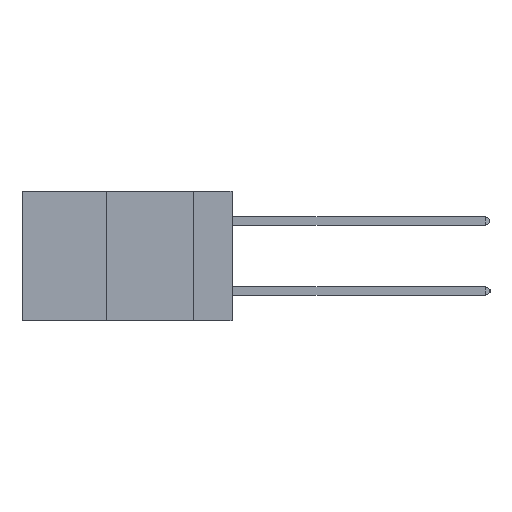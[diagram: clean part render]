
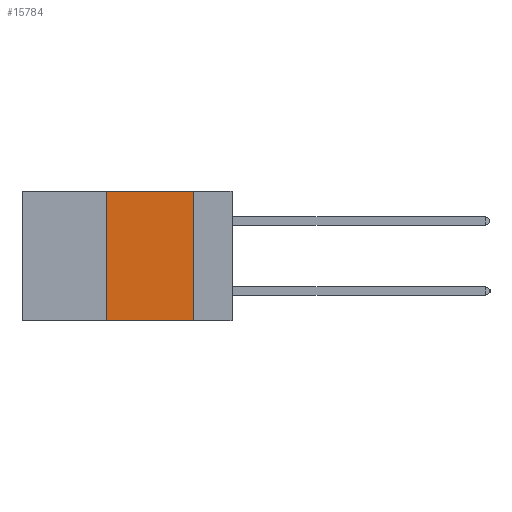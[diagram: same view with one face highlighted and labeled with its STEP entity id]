
A CAD part, left-side view. The second image highlights one B-rep face of the part: STEP entity #15784.
In plain terms, the highlighted planar face has unit normal (-1, 0, 0).
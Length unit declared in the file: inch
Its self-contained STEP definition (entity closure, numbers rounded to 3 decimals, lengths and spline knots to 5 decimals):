
#102 = DIRECTION ( 'NONE',  ( 0., 0., 1. ) ) ;
#830 = DIRECTION ( 'NONE',  ( 0., 0., -1. ) ) ;
#1790 = CARTESIAN_POINT ( 'NONE',  ( 0., 0.11, 0. ) ) ;
#1828 = VERTEX_POINT ( 'NONE', #8338 ) ;
#2219 = CARTESIAN_POINT ( 'NONE',  ( 0., 0.11, -0.37 ) ) ;
#2530 = DIRECTION ( 'NONE',  ( 1., 0., 0. ) ) ;
#2854 = PLANE ( 'NONE',  #9148 ) ;
#3167 = CARTESIAN_POINT ( 'NONE',  ( 0., 0.36, 0. ) ) ;
#4403 = DIRECTION ( 'NONE',  ( 0., 0., -1. ) ) ;
#4586 = ORIENTED_EDGE ( 'NONE', *, *, #15223, .F. ) ;
#4916 = EDGE_CURVE ( 'NONE', #12508, #11015, #20053, .T. ) ;
#5599 = LINE ( 'NONE', #16658, #7349 ) ;
#6593 = CARTESIAN_POINT ( 'NONE',  ( 0., 0.6, 0. ) ) ;
#7247 = DIRECTION ( 'NONE',  ( 0., -1., 0. ) ) ;
#7349 = VECTOR ( 'NONE', #7247, 39.37008 ) ;
#8008 = VECTOR ( 'NONE', #102, 39.37008 ) ;
#8338 = CARTESIAN_POINT ( 'NONE',  ( 0., 0.36, -0.37 ) ) ;
#8354 = VECTOR ( 'NONE', #830, 39.37008 ) ;
#9148 = AXIS2_PLACEMENT_3D ( 'NONE', #6593, #2530, #4403 ) ;
#9599 = ORIENTED_EDGE ( 'NONE', *, *, #10301, .F. ) ;
#10095 = LINE ( 'NONE', #23044, #8354 ) ;
#10301 = EDGE_CURVE ( 'NONE', #1828, #12508, #21917, .T. ) ;
#11015 = VERTEX_POINT ( 'NONE', #1790 ) ;
#11922 = VECTOR ( 'NONE', #23773, 39.37008 ) ;
#12042 = EDGE_CURVE ( 'NONE', #1828, #23139, #5599, .T. ) ;
#12508 = VERTEX_POINT ( 'NONE', #3167 ) ;
#15223 = EDGE_CURVE ( 'NONE', #11015, #23139, #10095, .T. ) ;
#15784 = ADVANCED_FACE ( 'NONE', ( #19367 ), #2854, .F. ) ;
#16475 = CARTESIAN_POINT ( 'NONE',  ( 0., 0.6, 0. ) ) ;
#16564 = EDGE_LOOP ( 'NONE', ( #4586, #17260, #9599, #19724 ) ) ;
#16658 = CARTESIAN_POINT ( 'NONE',  ( 0., 0.6, -0.37 ) ) ;
#17260 = ORIENTED_EDGE ( 'NONE', *, *, #4916, .F. ) ;
#19367 = FACE_OUTER_BOUND ( 'NONE', #16564, .T. ) ;
#19724 = ORIENTED_EDGE ( 'NONE', *, *, #12042, .T. ) ;
#20053 = LINE ( 'NONE', #16475, #11922 ) ;
#21917 = LINE ( 'NONE', #23944, #8008 ) ;
#23044 = CARTESIAN_POINT ( 'NONE',  ( 0., 0.11, 0. ) ) ;
#23139 = VERTEX_POINT ( 'NONE', #2219 ) ;
#23773 = DIRECTION ( 'NONE',  ( 0., -1., 0. ) ) ;
#23944 = CARTESIAN_POINT ( 'NONE',  ( 0., 0.36, 0. ) ) ;
